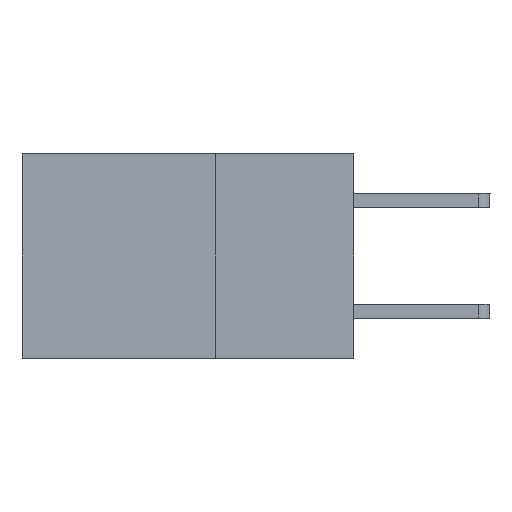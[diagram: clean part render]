
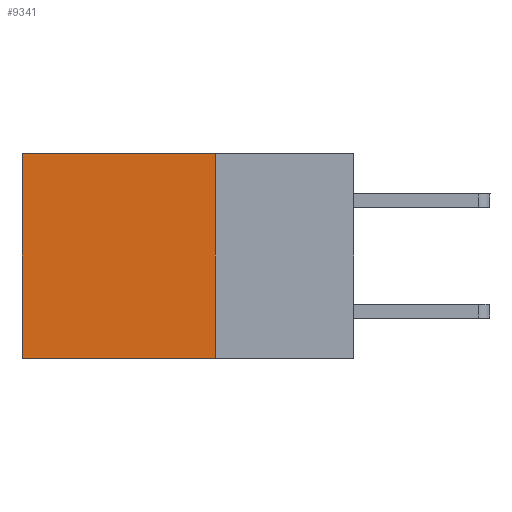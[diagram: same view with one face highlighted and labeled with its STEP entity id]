
A CAD part, left-side view. The second image highlights one B-rep face of the part: STEP entity #9341.
In plain terms, the highlighted planar face has unit normal (-1, 0, 0).
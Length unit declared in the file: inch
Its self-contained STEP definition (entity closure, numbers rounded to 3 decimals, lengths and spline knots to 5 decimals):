
#226 = CARTESIAN_POINT ( 'NONE',  ( 0.2875, 0.25, -0.37 ) ) ;
#475 = LINE ( 'NONE', #8669, #3504 ) ;
#566 = DIRECTION ( 'NONE',  ( 1., 0., 0. ) ) ;
#752 = CARTESIAN_POINT ( 'NONE',  ( 0.2875, 0.25, 0. ) ) ;
#1340 = VECTOR ( 'NONE', #1578, 39.37008 ) ;
#1377 = VERTEX_POINT ( 'NONE', #752 ) ;
#1578 = DIRECTION ( 'NONE',  ( 0., 0., -1. ) ) ;
#1920 = DIRECTION ( 'NONE',  ( 0., 1., 0. ) ) ;
#2292 = FACE_OUTER_BOUND ( 'NONE', #7626, .T. ) ;
#2429 = CARTESIAN_POINT ( 'NONE',  ( 0.2875, 0.6, -0.37 ) ) ;
#2598 = VECTOR ( 'NONE', #5966, 39.37008 ) ;
#3084 = CARTESIAN_POINT ( 'NONE',  ( 0.2875, 0.25, 0. ) ) ;
#3373 = LINE ( 'NONE', #5170, #2598 ) ;
#3504 = VECTOR ( 'NONE', #1920, 39.37008 ) ;
#3843 = PLANE ( 'NONE',  #9064 ) ;
#4362 = EDGE_CURVE ( 'NONE', #1377, #4411, #475, .T. ) ;
#4411 = VERTEX_POINT ( 'NONE', #8938 ) ;
#4782 = ORIENTED_EDGE ( 'NONE', *, *, #5875, .T. ) ;
#4785 = VECTOR ( 'NONE', #5182, 39.37008 ) ;
#4979 = VERTEX_POINT ( 'NONE', #226 ) ;
#5170 = CARTESIAN_POINT ( 'NONE',  ( 0.2875, 0.6, 0. ) ) ;
#5182 = DIRECTION ( 'NONE',  ( 0., 1., 0. ) ) ;
#5592 = LINE ( 'NONE', #3084, #1340 ) ;
#5875 = EDGE_CURVE ( 'NONE', #4411, #8347, #3373, .T. ) ;
#5966 = DIRECTION ( 'NONE',  ( 0., 0., -1. ) ) ;
#6160 = ORIENTED_EDGE ( 'NONE', *, *, #4362, .T. ) ;
#6840 = LINE ( 'NONE', #7762, #4785 ) ;
#7626 = EDGE_LOOP ( 'NONE', ( #4782, #8246, #9604, #6160 ) ) ;
#7762 = CARTESIAN_POINT ( 'NONE',  ( 0.2875, 0.25, -0.37 ) ) ;
#7853 = EDGE_CURVE ( 'NONE', #1377, #4979, #5592, .T. ) ;
#8246 = ORIENTED_EDGE ( 'NONE', *, *, #8570, .F. ) ;
#8347 = VERTEX_POINT ( 'NONE', #2429 ) ;
#8570 = EDGE_CURVE ( 'NONE', #4979, #8347, #6840, .T. ) ;
#8669 = CARTESIAN_POINT ( 'NONE',  ( 0.2875, 0.25, 0. ) ) ;
#8938 = CARTESIAN_POINT ( 'NONE',  ( 0.2875, 0.6, 0. ) ) ;
#9064 = AXIS2_PLACEMENT_3D ( 'NONE', #10238, #566, #9616 ) ;
#9341 = ADVANCED_FACE ( 'NONE', ( #2292 ), #3843, .F. ) ;
#9604 = ORIENTED_EDGE ( 'NONE', *, *, #7853, .F. ) ;
#9616 = DIRECTION ( 'NONE',  ( 0., 0., -1. ) ) ;
#10238 = CARTESIAN_POINT ( 'NONE',  ( 0.2875, 0.25, 0. ) ) ;
